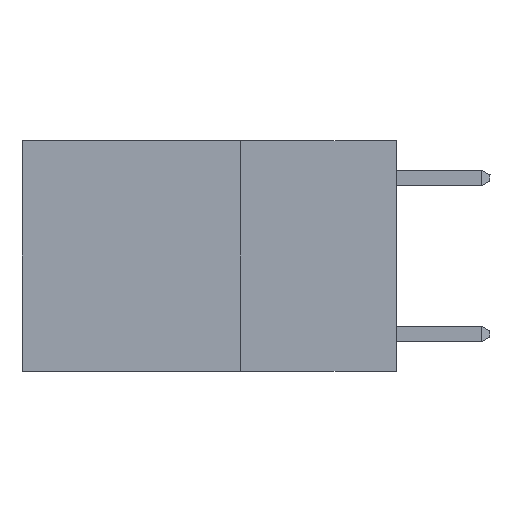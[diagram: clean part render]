
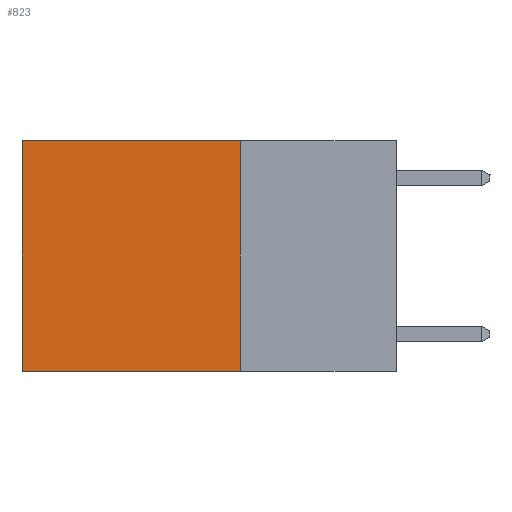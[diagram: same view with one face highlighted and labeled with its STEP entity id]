
A CAD part, left-side view. The second image highlights one B-rep face of the part: STEP entity #823.
In plain terms, the highlighted planar face has unit normal (-1, 0, 0).
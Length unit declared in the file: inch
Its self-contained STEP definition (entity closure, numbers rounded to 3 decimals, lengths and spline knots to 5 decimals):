
#451 = VECTOR ( 'NONE', #14780, 39.37008 ) ;
#823 = ADVANCED_FACE ( 'NONE', ( #23214 ), #8163, .F. ) ;
#1869 = VERTEX_POINT ( 'NONE', #18584 ) ;
#2401 = DIRECTION ( 'NONE',  ( 0., 0., -1. ) ) ;
#5206 = CARTESIAN_POINT ( 'NONE',  ( 0.2625, 0.25, 0. ) ) ;
#5872 = VECTOR ( 'NONE', #17568, 39.37008 ) ;
#6750 = CARTESIAN_POINT ( 'NONE',  ( 0.2625, 0.6, -0.37 ) ) ;
#6907 = DIRECTION ( 'NONE',  ( 0., 1., 0. ) ) ;
#7124 = LINE ( 'NONE', #16525, #451 ) ;
#7794 = ORIENTED_EDGE ( 'NONE', *, *, #8044, .F. ) ;
#8044 = EDGE_CURVE ( 'NONE', #17380, #11722, #22104, .T. ) ;
#8052 = CARTESIAN_POINT ( 'NONE',  ( 0.2625, 0.25, 0. ) ) ;
#8163 = PLANE ( 'NONE',  #11168 ) ;
#9048 = CARTESIAN_POINT ( 'NONE',  ( 0.2625, 0.25, -0.37 ) ) ;
#9536 = CARTESIAN_POINT ( 'NONE',  ( 0.2625, 0.6, 0. ) ) ;
#11005 = DIRECTION ( 'NONE',  ( 0., 1., 0. ) ) ;
#11168 = AXIS2_PLACEMENT_3D ( 'NONE', #8052, #22967, #2401 ) ;
#11722 = VERTEX_POINT ( 'NONE', #6750 ) ;
#13018 = ORIENTED_EDGE ( 'NONE', *, *, #19945, .T. ) ;
#13736 = CARTESIAN_POINT ( 'NONE',  ( 0.2625, 0.6, 0. ) ) ;
#13911 = CARTESIAN_POINT ( 'NONE',  ( 0.2625, 0.25, -0.37 ) ) ;
#14750 = ORIENTED_EDGE ( 'NONE', *, *, #18962, .T. ) ;
#14780 = DIRECTION ( 'NONE',  ( 0., 0., -1. ) ) ;
#16525 = CARTESIAN_POINT ( 'NONE',  ( 0.2625, 0.25, 0. ) ) ;
#17380 = VERTEX_POINT ( 'NONE', #13911 ) ;
#17568 = DIRECTION ( 'NONE',  ( 0., 0., -1. ) ) ;
#18584 = CARTESIAN_POINT ( 'NONE',  ( 0.2625, 0.25, 0. ) ) ;
#18822 = ORIENTED_EDGE ( 'NONE', *, *, #24744, .F. ) ;
#18962 = EDGE_CURVE ( 'NONE', #1869, #20367, #22416, .T. ) ;
#19744 = EDGE_LOOP ( 'NONE', ( #13018, #7794, #18822, #14750 ) ) ;
#19945 = EDGE_CURVE ( 'NONE', #20367, #11722, #21210, .T. ) ;
#20367 = VERTEX_POINT ( 'NONE', #13736 ) ;
#20569 = VECTOR ( 'NONE', #6907, 39.37008 ) ;
#20607 = VECTOR ( 'NONE', #11005, 39.37008 ) ;
#21210 = LINE ( 'NONE', #9536, #5872 ) ;
#22104 = LINE ( 'NONE', #9048, #20569 ) ;
#22416 = LINE ( 'NONE', #5206, #20607 ) ;
#22967 = DIRECTION ( 'NONE',  ( 1., 0., 0. ) ) ;
#23214 = FACE_OUTER_BOUND ( 'NONE', #19744, .T. ) ;
#24744 = EDGE_CURVE ( 'NONE', #1869, #17380, #7124, .T. ) ;
